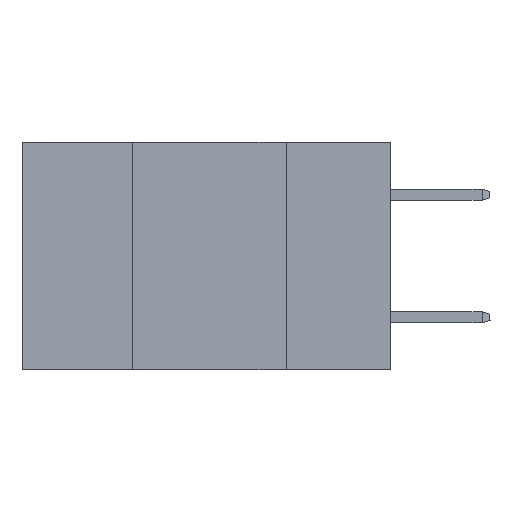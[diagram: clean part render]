
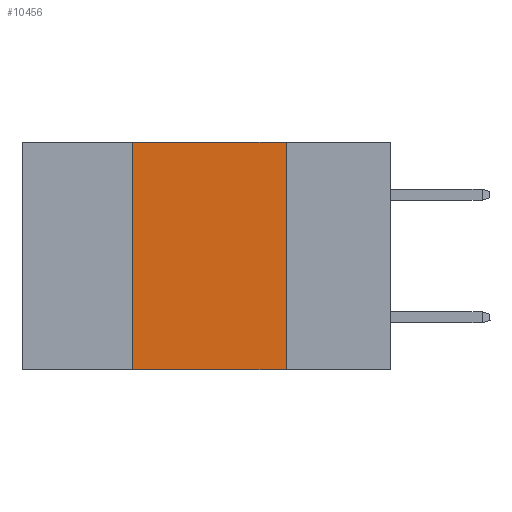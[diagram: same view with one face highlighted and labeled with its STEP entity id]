
A CAD part, left-side view. The second image highlights one B-rep face of the part: STEP entity #10456.
In plain terms, the highlighted planar face has unit normal (-1, 0, 0).
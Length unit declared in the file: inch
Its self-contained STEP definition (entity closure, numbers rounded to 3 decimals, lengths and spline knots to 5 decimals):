
#380 = CARTESIAN_POINT ( 'NONE',  ( 0., 0.6, -0.37 ) ) ;
#407 = CARTESIAN_POINT ( 'NONE',  ( 0., 0.42, 0. ) ) ;
#887 = VERTEX_POINT ( 'NONE', #9101 ) ;
#1011 = ORIENTED_EDGE ( 'NONE', *, *, #10173, .F. ) ;
#1139 = CARTESIAN_POINT ( 'NONE',  ( 0., 0.17, 0. ) ) ;
#2190 = LINE ( 'NONE', #380, #11169 ) ;
#2291 = DIRECTION ( 'NONE',  ( 0., -1., 0. ) ) ;
#2488 = EDGE_LOOP ( 'NONE', ( #3765, #1011, #4369, #9933 ) ) ;
#2683 = DIRECTION ( 'NONE',  ( 0., -1., 0. ) ) ;
#2820 = CARTESIAN_POINT ( 'NONE',  ( 0., 0.17, -0.37 ) ) ;
#2912 = LINE ( 'NONE', #8543, #3483 ) ;
#3096 = CARTESIAN_POINT ( 'NONE',  ( 0., 0.6, 0. ) ) ;
#3177 = DIRECTION ( 'NONE',  ( 0., 0., 1. ) ) ;
#3483 = VECTOR ( 'NONE', #3177, 39.37008 ) ;
#3765 = ORIENTED_EDGE ( 'NONE', *, *, #11101, .F. ) ;
#4369 = ORIENTED_EDGE ( 'NONE', *, *, #10516, .F. ) ;
#4939 = DIRECTION ( 'NONE',  ( 0., 0., -1. ) ) ;
#5753 = DIRECTION ( 'NONE',  ( 0., 0., -1. ) ) ;
#6121 = CARTESIAN_POINT ( 'NONE',  ( 0., 0.17, 0. ) ) ;
#6335 = LINE ( 'NONE', #8095, #11014 ) ;
#8095 = CARTESIAN_POINT ( 'NONE',  ( 0., 0.6, 0. ) ) ;
#8269 = FACE_OUTER_BOUND ( 'NONE', #2488, .T. ) ;
#8316 = AXIS2_PLACEMENT_3D ( 'NONE', #3096, #10244, #4939 ) ;
#8472 = PLANE ( 'NONE',  #8316 ) ;
#8543 = CARTESIAN_POINT ( 'NONE',  ( 0., 0.42, 0. ) ) ;
#8659 = VECTOR ( 'NONE', #5753, 39.37008 ) ;
#8938 = LINE ( 'NONE', #1139, #8659 ) ;
#9101 = CARTESIAN_POINT ( 'NONE',  ( 0., 0.42, -0.37 ) ) ;
#9911 = EDGE_CURVE ( 'NONE', #887, #11682, #2190, .T. ) ;
#9933 = ORIENTED_EDGE ( 'NONE', *, *, #9911, .T. ) ;
#10173 = EDGE_CURVE ( 'NONE', #10585, #10678, #6335, .T. ) ;
#10244 = DIRECTION ( 'NONE',  ( 1., 0., 0. ) ) ;
#10456 = ADVANCED_FACE ( 'NONE', ( #8269 ), #8472, .F. ) ;
#10516 = EDGE_CURVE ( 'NONE', #887, #10585, #2912, .T. ) ;
#10585 = VERTEX_POINT ( 'NONE', #407 ) ;
#10678 = VERTEX_POINT ( 'NONE', #6121 ) ;
#11014 = VECTOR ( 'NONE', #2683, 39.37008 ) ;
#11101 = EDGE_CURVE ( 'NONE', #10678, #11682, #8938, .T. ) ;
#11169 = VECTOR ( 'NONE', #2291, 39.37008 ) ;
#11682 = VERTEX_POINT ( 'NONE', #2820 ) ;
